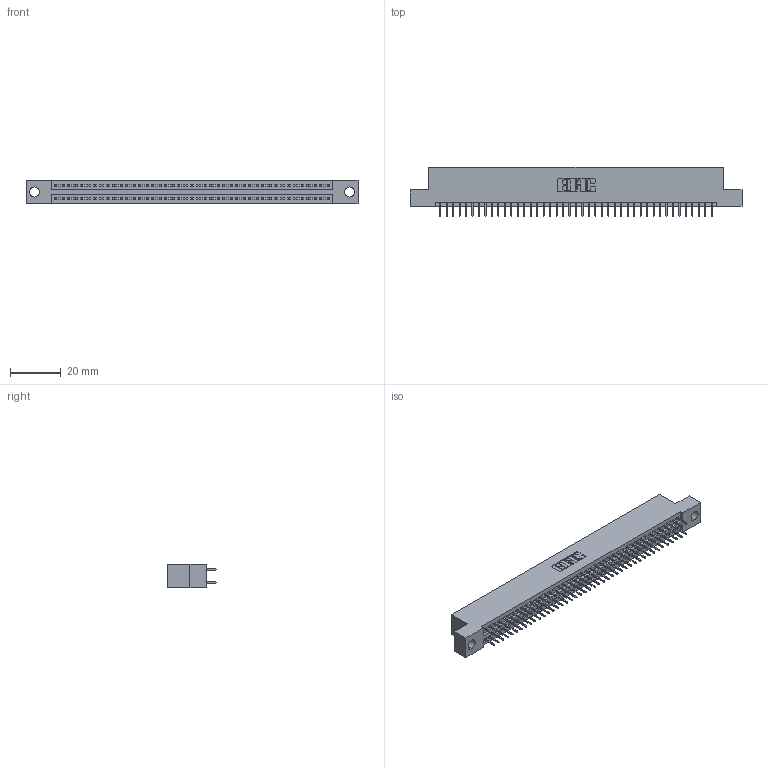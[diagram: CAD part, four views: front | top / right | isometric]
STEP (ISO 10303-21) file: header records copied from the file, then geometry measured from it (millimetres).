
FILE_DESCRIPTION (( 'STEP AP203' ), '1' );
FILE_NAME ('345-086-524-204.STEP', '2021-05-20T13:20:09', ( '' ), ( '' ), 'SwSTEP 2.0', 'SolidWorks 2020', '' );
FILE_SCHEMA (( 'CONFIG_CONTROL_DESIGN' ));
Length unit declared in the file: inch
Products named in the file (3): 345 Part_Flush Mounting Lugs - 0.156 Dia-TI; 345-086-524-204; 345-292-001_345-293-124
Assembly tree (87 placements, depth 2):
  345-086-524-204
    345 Part_Flush Mounting Lugs - 0.156 Dia-TI
    345-292-001_345-293-124  x86
Bounding box: 130.43 x 19.35 x 9.4 mm (x, y, z)
Volume: 12443.2 mm3; surface area: 17920.5 mm2
Topology: 87 solids, 87 shells, 4784 faces, 13535 edges, 8678 vertices
Faces by surface type: plane 3448, cylinder 1336
Entity records: 34097 total; most frequent: CARTESIAN_POINT 5718, ORIENTED_EDGE 5650, DIRECTION 5041, EDGE_CURVE 2825, LINE 2525, VECTOR 2525, VERTEX_POINT 1878, AXIS2_PLACEMENT_3D 1258
